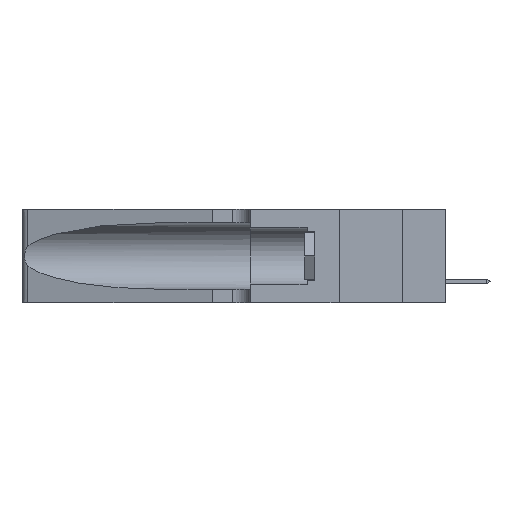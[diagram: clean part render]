
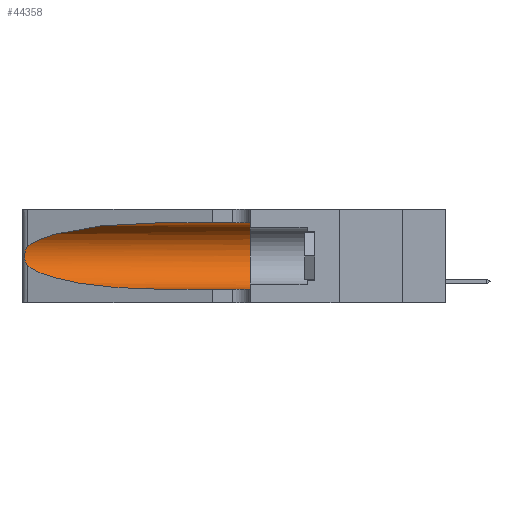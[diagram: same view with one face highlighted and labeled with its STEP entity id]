
A CAD part, left-side view. The second image highlights one B-rep face of the part: STEP entity #44358.
In plain terms, the highlighted cylindrical face has radius 3.308 mm (diameter 6.617 mm), a partial arc.
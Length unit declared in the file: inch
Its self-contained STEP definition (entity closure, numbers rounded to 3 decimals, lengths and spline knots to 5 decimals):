
#126 = EDGE_CURVE ( 'NONE', #28513, #9824, #43411, .T. ) ;
#219 = ORIENTED_EDGE ( 'NONE', *, *, #126, .F. ) ;
#1471 = CARTESIAN_POINT ( 'NONE',  ( 0.25789, 1.23486, 0.15765 ) ) ;
#2022 = CARTESIAN_POINT ( 'NONE',  ( 0.25487, 1.22718, 0.22369 ) ) ;
#2384 = VERTEX_POINT ( 'NONE', #28011 ) ;
#2958 = VECTOR ( 'NONE', #28948, 39.37008 ) ;
#6525 = CARTESIAN_POINT ( 'NONE',  ( 0.26075, 1.23896, 0.19203 ) ) ;
#7126 = CARTESIAN_POINT ( 'NONE',  ( 0.25639, 1.23184, 0.21858 ) ) ;
#9009 = VERTEX_POINT ( 'NONE', #39211 ) ;
#9591 = VECTOR ( 'NONE', #31278, 39.37008 ) ;
#9657 = FACE_OUTER_BOUND ( 'NONE', #35522, .T. ) ;
#9824 = VERTEX_POINT ( 'NONE', #35705 ) ;
#11647 = B_SPLINE_CURVE_WITH_KNOTS ( 'NONE', 3,
 ( #2022, #30205, #7126, #12835, #25456, #33480, #6525, #33132, #31390, #16852, #1471, #22795, #31039, #34440 ),
 .UNSPECIFIED., .F., .F.,
 ( 4, 2, 2, 2, 2, 2, 4 ),
 ( 0., 0.00027, 0.00053, 0.00107, 0.0016, 0.00187, 0.00214 ),
 .UNSPECIFIED. ) ;
#12498 =( BOUNDED_CURVE ( )  B_SPLINE_CURVE ( 3, ( #23661, #43309, #42987, #39305 ),
 .UNSPECIFIED., .F., .T. ) 
 B_SPLINE_CURVE_WITH_KNOTS ( ( 4, 4 ),
 ( 3.44316, 4.71239 ),
 .UNSPECIFIED. ) 
 CURVE ( )  GEOMETRIC_REPRESENTATION_ITEM ( )  RATIONAL_B_SPLINE_CURVE ( ( 1., 0.87, 0.87, 1. ) ) 
 REPRESENTATION_ITEM ( '' )  );
#12835 = CARTESIAN_POINT ( 'NONE',  ( 0.25787, 1.23484, 0.2124 ) ) ;
#14784 = EDGE_CURVE ( 'NONE', #36788, #2384, #11647, .T. ) ;
#15988 = CARTESIAN_POINT ( 'NONE',  ( 0.1305, 1.61858, 0.31525 ) ) ;
#16685 = DIRECTION ( 'NONE',  ( 0., 0., 1. ) ) ;
#16852 = CARTESIAN_POINT ( 'NONE',  ( 0.25856, 1.23593, 0.16098 ) ) ;
#16930 = DIRECTION ( 'NONE',  ( 0., -1., 0. ) ) ;
#17426 = CARTESIAN_POINT ( 'NONE',  ( 0.1305, 1.61858, 0.05475 ) ) ;
#18038 = ORIENTED_EDGE ( 'NONE', *, *, #32574, .T. ) ;
#22011 = LINE ( 'NONE', #17426, #2958 ) ;
#22236 = ORIENTED_EDGE ( 'NONE', *, *, #14784, .T. ) ;
#22795 = CARTESIAN_POINT ( 'NONE',  ( 0.25639, 1.23186, 0.15144 ) ) ;
#23656 = CARTESIAN_POINT ( 'NONE',  ( 0.25487, 1.22718, 0.22369 ) ) ;
#23661 = CARTESIAN_POINT ( 'NONE',  ( 0.25487, 1.22718, 0.14631 ) ) ;
#24520 = CARTESIAN_POINT ( 'NONE',  ( 0.1305, 0.35, 0.185 ) ) ;
#24766 = ORIENTED_EDGE ( 'NONE', *, *, #35054, .F. ) ;
#25456 = CARTESIAN_POINT ( 'NONE',  ( 0.25854, 1.2359, 0.20912 ) ) ;
#25469 = EDGE_CURVE ( 'NONE', #26267, #9824, #22011, .T. ) ;
#26112 = AXIS2_PLACEMENT_3D ( 'NONE', #24520, #47661, #16685 ) ;
#26267 = VERTEX_POINT ( 'NONE', #30403 ) ;
#26305 = AXIS2_PLACEMENT_3D ( 'NONE', #43418, #16930, #28451 ) ;
#26413 = CARTESIAN_POINT ( 'NONE',  ( 0.25487, 1.22718, 0.22369 ) ) ;
#28011 = CARTESIAN_POINT ( 'NONE',  ( 0.25487, 1.22718, 0.14631 ) ) ;
#28451 = DIRECTION ( 'NONE',  ( 0., 0., -1. ) ) ;
#28513 = VERTEX_POINT ( 'NONE', #41644 ) ;
#28816 = EDGE_CURVE ( 'NONE', #2384, #26267, #12498, .T. ) ;
#28948 = DIRECTION ( 'NONE',  ( 0., -1., 0. ) ) ;
#29232 = CARTESIAN_POINT ( 'NONE',  ( 0.18966, 0.96281, 0.31525 ) ) ;
#30205 = CARTESIAN_POINT ( 'NONE',  ( 0.25555, 1.22994, 0.2215 ) ) ;
#30403 = CARTESIAN_POINT ( 'NONE',  ( 0.1305, 0.72297, 0.05475 ) ) ;
#31039 = CARTESIAN_POINT ( 'NONE',  ( 0.25555, 1.22993, 0.14849 ) ) ;
#31278 = DIRECTION ( 'NONE',  ( 0., -1., 0. ) ) ;
#31378 = ORIENTED_EDGE ( 'NONE', *, *, #28816, .T. ) ;
#31390 = CARTESIAN_POINT ( 'NONE',  ( 0.26017, 1.23833, 0.17102 ) ) ;
#32574 = EDGE_CURVE ( 'NONE', #9009, #36788, #38308, .T. ) ;
#33132 = CARTESIAN_POINT ( 'NONE',  ( 0.26075, 1.23896, 0.178 ) ) ;
#33480 = CARTESIAN_POINT ( 'NONE',  ( 0.26018, 1.23835, 0.19895 ) ) ;
#34440 = CARTESIAN_POINT ( 'NONE',  ( 0.25487, 1.22718, 0.14631 ) ) ;
#34571 = CARTESIAN_POINT ( 'NONE',  ( 0.2373, 1.15595, 0.28018 ) ) ;
#35054 = EDGE_CURVE ( 'NONE', #9009, #28513, #47248, .T. ) ;
#35522 = EDGE_LOOP ( 'NONE', ( #18038, #22236, #31378, #47673, #219, #24766 ) ) ;
#35705 = CARTESIAN_POINT ( 'NONE',  ( 0.1305, 0.35, 0.05475 ) ) ;
#36788 = VERTEX_POINT ( 'NONE', #23656 ) ;
#38308 =( BOUNDED_CURVE ( )  B_SPLINE_CURVE ( 3, ( #40689, #29232, #34571, #26413 ),
 .UNSPECIFIED., .F., .T. ) 
 B_SPLINE_CURVE_WITH_KNOTS ( ( 4, 4 ),
 ( 1.5708, 2.84003 ),
 .UNSPECIFIED. ) 
 CURVE ( )  GEOMETRIC_REPRESENTATION_ITEM ( )  RATIONAL_B_SPLINE_CURVE ( ( 1., 0.87, 0.87, 1. ) ) 
 REPRESENTATION_ITEM ( '' )  );
#39211 = CARTESIAN_POINT ( 'NONE',  ( 0.1305, 0.72297, 0.31525 ) ) ;
#39305 = CARTESIAN_POINT ( 'NONE',  ( 0.1305, 0.72297, 0.05475 ) ) ;
#40689 = CARTESIAN_POINT ( 'NONE',  ( 0.1305, 0.72297, 0.31525 ) ) ;
#41644 = CARTESIAN_POINT ( 'NONE',  ( 0.1305, 0.35, 0.31525 ) ) ;
#42987 = CARTESIAN_POINT ( 'NONE',  ( 0.18966, 0.96281, 0.05475 ) ) ;
#43309 = CARTESIAN_POINT ( 'NONE',  ( 0.2373, 1.15595, 0.08982 ) ) ;
#43411 = CIRCLE ( 'NONE', #26112, 0.13025 ) ;
#43418 = CARTESIAN_POINT ( 'NONE',  ( 0.1305, 1.61858, 0.185 ) ) ;
#44358 = ADVANCED_FACE ( 'NONE', ( #9657 ), #46695, .F. ) ;
#46695 = CYLINDRICAL_SURFACE ( 'NONE', #26305, 0.13025 ) ;
#47248 = LINE ( 'NONE', #15988, #9591 ) ;
#47661 = DIRECTION ( 'NONE',  ( 0., 1., 0. ) ) ;
#47673 = ORIENTED_EDGE ( 'NONE', *, *, #25469, .T. ) ;
